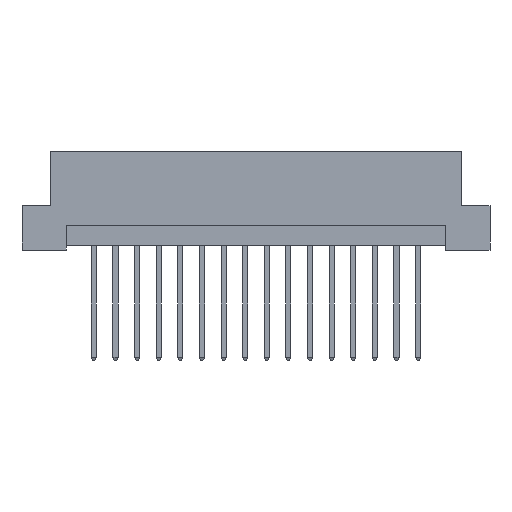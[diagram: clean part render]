
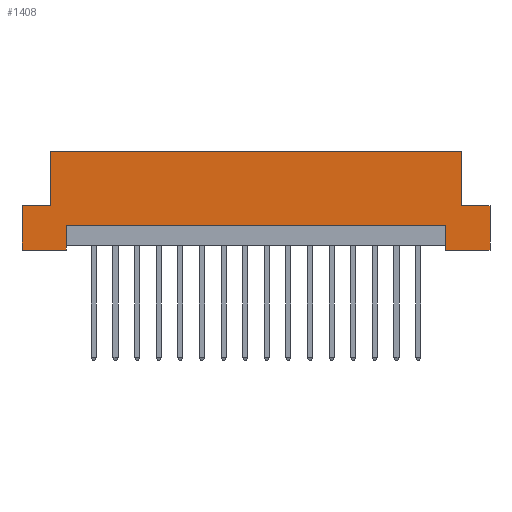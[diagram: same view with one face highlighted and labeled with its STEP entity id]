
A CAD part, front view. The second image highlights one B-rep face of the part: STEP entity #1408.
In plain terms, the highlighted planar face has unit normal (0, -1, 0).
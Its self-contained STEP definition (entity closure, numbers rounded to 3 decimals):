
#46 = CARTESIAN_POINT ( 'NONE',  ( -27.5, 0., 0. ) ) ;
#369 = VECTOR ( 'NONE', #6360, 1000. ) ;
#598 = CARTESIAN_POINT ( 'NONE',  ( -24.2, 0., 5.2 ) ) ;
#704 = LINE ( 'NONE', #9031, #6258 ) ;
#716 = VECTOR ( 'NONE', #5039, 1000. ) ;
#936 = DIRECTION ( 'NONE',  ( 0., 0., -1. ) ) ;
#1008 = DIRECTION ( 'NONE',  ( 0., 0., 1. ) ) ;
#1187 = VECTOR ( 'NONE', #2690, 1000. ) ;
#1259 = EDGE_CURVE ( 'NONE', #2674, #9068, #9768, .T. ) ;
#1408 = ADVANCED_FACE ( 'NONE', ( #3281 ), #1703, .F. ) ;
#1536 = DIRECTION ( 'NONE',  ( 1., 0., 0. ) ) ;
#1653 = VECTOR ( 'NONE', #936, 1000. ) ;
#1656 = AXIS2_PLACEMENT_3D ( 'NONE', #8571, #9326, #6177 ) ;
#1703 = PLANE ( 'NONE',  #1656 ) ;
#1706 = VERTEX_POINT ( 'NONE', #6761 ) ;
#1828 = VECTOR ( 'NONE', #6589, 1000. ) ;
#1883 = LINE ( 'NONE', #7255, #7709 ) ;
#1936 = LINE ( 'NONE', #8755, #1187 ) ;
#1980 = EDGE_CURVE ( 'NONE', #2625, #8706, #6359, .T. ) ;
#2163 = CARTESIAN_POINT ( 'NONE',  ( -22.3, 0., 2.9 ) ) ;
#2541 = LINE ( 'NONE', #9364, #6823 ) ;
#2558 = VERTEX_POINT ( 'NONE', #5583 ) ;
#2625 = VERTEX_POINT ( 'NONE', #9041 ) ;
#2674 = VERTEX_POINT ( 'NONE', #6640 ) ;
#2690 = DIRECTION ( 'NONE',  ( 1., 0., 0. ) ) ;
#2909 = ORIENTED_EDGE ( 'NONE', *, *, #4452, .F. ) ;
#2931 = LINE ( 'NONE', #5301, #9353 ) ;
#2935 = CARTESIAN_POINT ( 'NONE',  ( -27.5, 0., 5.2 ) ) ;
#3127 = EDGE_CURVE ( 'NONE', #7180, #1706, #2931, .T. ) ;
#3133 = ORIENTED_EDGE ( 'NONE', *, *, #1980, .F. ) ;
#3193 = ORIENTED_EDGE ( 'NONE', *, *, #9565, .F. ) ;
#3281 = FACE_OUTER_BOUND ( 'NONE', #8774, .T. ) ;
#3323 = CARTESIAN_POINT ( 'NONE',  ( -27.5, 0., 0. ) ) ;
#3803 = EDGE_CURVE ( 'NONE', #2625, #6923, #4646, .T. ) ;
#4004 = ORIENTED_EDGE ( 'NONE', *, *, #3803, .T. ) ;
#4257 = CARTESIAN_POINT ( 'NONE',  ( 22.3, 0., 2.9 ) ) ;
#4452 = EDGE_CURVE ( 'NONE', #9098, #7180, #7839, .T. ) ;
#4602 = ORIENTED_EDGE ( 'NONE', *, *, #5733, .F. ) ;
#4646 = LINE ( 'NONE', #6203, #5990 ) ;
#4689 = LINE ( 'NONE', #9553, #1828 ) ;
#4751 = CARTESIAN_POINT ( 'NONE',  ( -22.3, 0., 0.5 ) ) ;
#4782 = CARTESIAN_POINT ( 'NONE',  ( -22.3, 0., 0. ) ) ;
#5036 = VECTOR ( 'NONE', #1008, 1000. ) ;
#5039 = DIRECTION ( 'NONE',  ( -1., 0., 0. ) ) ;
#5129 = VECTOR ( 'NONE', #9077, 1000. ) ;
#5301 = CARTESIAN_POINT ( 'NONE',  ( -27.5, 0., 11.6 ) ) ;
#5332 = CARTESIAN_POINT ( 'NONE',  ( -24.2, 0., 11.6 ) ) ;
#5360 = EDGE_CURVE ( 'NONE', #8706, #8415, #7808, .T. ) ;
#5490 = ORIENTED_EDGE ( 'NONE', *, *, #6921, .F. ) ;
#5583 = CARTESIAN_POINT ( 'NONE',  ( 27.5, 0., 0. ) ) ;
#5733 = EDGE_CURVE ( 'NONE', #5861, #6562, #704, .T. ) ;
#5861 = VERTEX_POINT ( 'NONE', #7878 ) ;
#5990 = VECTOR ( 'NONE', #6245, 1000. ) ;
#6023 = DIRECTION ( 'NONE',  ( 1., 0., 0. ) ) ;
#6177 = DIRECTION ( 'NONE',  ( 0., 0., 1. ) ) ;
#6203 = CARTESIAN_POINT ( 'NONE',  ( 22.3, 0., 0.5 ) ) ;
#6223 = ORIENTED_EDGE ( 'NONE', *, *, #8474, .F. ) ;
#6245 = DIRECTION ( 'NONE',  ( 0., 0., -1. ) ) ;
#6258 = VECTOR ( 'NONE', #6023, 1000. ) ;
#6280 = ORIENTED_EDGE ( 'NONE', *, *, #7938, .T. ) ;
#6359 = LINE ( 'NONE', #4257, #716 ) ;
#6360 = DIRECTION ( 'NONE',  ( -1., 0., 0. ) ) ;
#6562 = VERTEX_POINT ( 'NONE', #9707 ) ;
#6589 = DIRECTION ( 'NONE',  ( -1., 0., 0. ) ) ;
#6640 = CARTESIAN_POINT ( 'NONE',  ( -27.5, 0., 0. ) ) ;
#6761 = CARTESIAN_POINT ( 'NONE',  ( 24.2, 0., 11.6 ) ) ;
#6797 = CARTESIAN_POINT ( 'NONE',  ( 22.3, 0., 0. ) ) ;
#6823 = VECTOR ( 'NONE', #8557, 1000. ) ;
#6882 = EDGE_CURVE ( 'NONE', #9068, #9098, #1936, .T. ) ;
#6921 = EDGE_CURVE ( 'NONE', #6562, #2558, #1883, .T. ) ;
#6923 = VERTEX_POINT ( 'NONE', #6797 ) ;
#7109 = LINE ( 'NONE', #3323, #369 ) ;
#7180 = VERTEX_POINT ( 'NONE', #5332 ) ;
#7255 = CARTESIAN_POINT ( 'NONE',  ( 27.5, 0., 0. ) ) ;
#7709 = VECTOR ( 'NONE', #8336, 1000. ) ;
#7808 = LINE ( 'NONE', #4751, #1653 ) ;
#7839 = LINE ( 'NONE', #7887, #5036 ) ;
#7842 = ORIENTED_EDGE ( 'NONE', *, *, #5360, .F. ) ;
#7878 = CARTESIAN_POINT ( 'NONE',  ( 24.2, 0., 5.2 ) ) ;
#7887 = CARTESIAN_POINT ( 'NONE',  ( -24.2, 0., 5.2 ) ) ;
#7938 = EDGE_CURVE ( 'NONE', #5861, #1706, #2541, .T. ) ;
#8051 = ORIENTED_EDGE ( 'NONE', *, *, #3127, .F. ) ;
#8336 = DIRECTION ( 'NONE',  ( 0., 0., -1. ) ) ;
#8415 = VERTEX_POINT ( 'NONE', #4782 ) ;
#8474 = EDGE_CURVE ( 'NONE', #8415, #2674, #4689, .T. ) ;
#8557 = DIRECTION ( 'NONE',  ( 0., 0., 1. ) ) ;
#8571 = CARTESIAN_POINT ( 'NONE',  ( -27.5, 0., 11.6 ) ) ;
#8706 = VERTEX_POINT ( 'NONE', #2163 ) ;
#8755 = CARTESIAN_POINT ( 'NONE',  ( -27.5, 0., 5.2 ) ) ;
#8774 = EDGE_LOOP ( 'NONE', ( #3133, #4004, #3193, #5490, #4602, #6280, #8051, #2909, #9052, #9012, #6223, #7842 ) ) ;
#9012 = ORIENTED_EDGE ( 'NONE', *, *, #1259, .F. ) ;
#9031 = CARTESIAN_POINT ( 'NONE',  ( 27.5, 0., 5.2 ) ) ;
#9041 = CARTESIAN_POINT ( 'NONE',  ( 22.3, 0., 2.9 ) ) ;
#9052 = ORIENTED_EDGE ( 'NONE', *, *, #6882, .F. ) ;
#9068 = VERTEX_POINT ( 'NONE', #2935 ) ;
#9077 = DIRECTION ( 'NONE',  ( 0., 0., 1. ) ) ;
#9098 = VERTEX_POINT ( 'NONE', #598 ) ;
#9326 = DIRECTION ( 'NONE',  ( 0., 1., 0. ) ) ;
#9353 = VECTOR ( 'NONE', #1536, 1000. ) ;
#9364 = CARTESIAN_POINT ( 'NONE',  ( 24.2, 0., 5.2 ) ) ;
#9553 = CARTESIAN_POINT ( 'NONE',  ( -27.5, 0., 0. ) ) ;
#9565 = EDGE_CURVE ( 'NONE', #2558, #6923, #7109, .T. ) ;
#9707 = CARTESIAN_POINT ( 'NONE',  ( 27.5, 0., 5.2 ) ) ;
#9768 = LINE ( 'NONE', #46, #5129 ) ;
